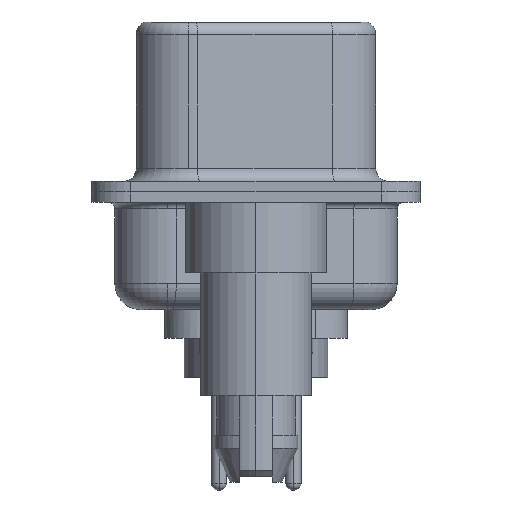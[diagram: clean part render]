
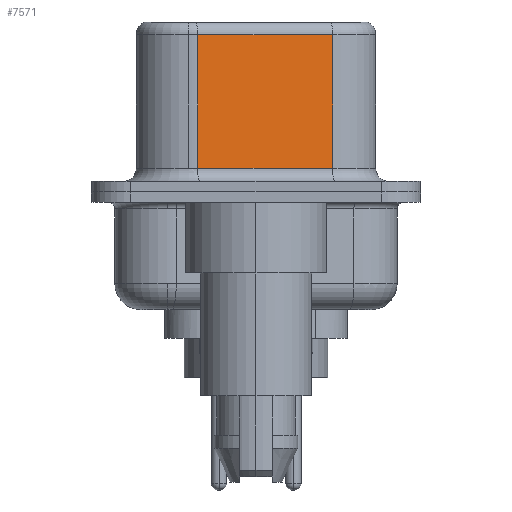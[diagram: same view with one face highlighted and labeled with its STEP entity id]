
A CAD part, left-side view. The second image highlights one B-rep face of the part: STEP entity #7571.
In plain terms, the highlighted planar face has unit normal (-0.985, -0.174, 0).
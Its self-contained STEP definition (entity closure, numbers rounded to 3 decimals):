
#718 = DIRECTION ( 'NONE',  ( 0., 0., -1. ) ) ;
#1950 = FACE_OUTER_BOUND ( 'NONE', #14733, .T. ) ;
#5108 = DIRECTION ( 'NONE',  ( -0.174, 0.985, 0. ) ) ;
#5463 = CARTESIAN_POINT ( 'NONE',  ( 4.58, -2.927, 0.9 ) ) ;
#5551 = CARTESIAN_POINT ( 'NONE',  ( 4.58, -2.927, 6.02 ) ) ;
#5612 = CARTESIAN_POINT ( 'NONE',  ( 4.58, -2.927, 6.02 ) ) ;
#6773 = VERTEX_POINT ( 'NONE', #5463 ) ;
#7039 = VERTEX_POINT ( 'NONE', #9002 ) ;
#7060 = DIRECTION ( 'NONE',  ( -0.174, 0.985, 0. ) ) ;
#7571 = ADVANCED_FACE ( 'NONE', ( #1950 ), #9399, .F. ) ;
#7811 = EDGE_CURVE ( 'NONE', #7039, #6773, #18312, .T. ) ;
#8519 = CARTESIAN_POINT ( 'NONE',  ( 3.67, 2.233, 6.52 ) ) ;
#9002 = CARTESIAN_POINT ( 'NONE',  ( 3.67, 2.233, 0.9 ) ) ;
#9286 = ORIENTED_EDGE ( 'NONE', *, *, #13643, .T. ) ;
#9399 = PLANE ( 'NONE',  #19000 ) ;
#9784 = ORIENTED_EDGE ( 'NONE', *, *, #12099, .F. ) ;
#9889 = DIRECTION ( 'NONE',  ( 0.174, -0.985, 0. ) ) ;
#10787 = ORIENTED_EDGE ( 'NONE', *, *, #7811, .T. ) ;
#10982 = CARTESIAN_POINT ( 'NONE',  ( 4.58, -2.927, 6.52 ) ) ;
#11325 = LINE ( 'NONE', #5612, #18797 ) ;
#11438 = VECTOR ( 'NONE', #17360, 1000. ) ;
#11714 = LINE ( 'NONE', #10982, #15245 ) ;
#11905 = LINE ( 'NONE', #8519, #11438 ) ;
#12099 = EDGE_CURVE ( 'NONE', #17632, #6773, #11714, .T. ) ;
#13347 = ORIENTED_EDGE ( 'NONE', *, *, #18717, .T. ) ;
#13643 = EDGE_CURVE ( 'NONE', #17560, #7039, #11905, .T. ) ;
#13933 = DIRECTION ( 'NONE',  ( 0.985, 0.174, 0. ) ) ;
#14363 = CARTESIAN_POINT ( 'NONE',  ( 4.58, -2.927, 0.9 ) ) ;
#14435 = VECTOR ( 'NONE', #9889, 1000. ) ;
#14733 = EDGE_LOOP ( 'NONE', ( #9784, #13347, #9286, #10787 ) ) ;
#15245 = VECTOR ( 'NONE', #718, 1000. ) ;
#15326 = CARTESIAN_POINT ( 'NONE',  ( 4.58, -2.927, 6.52 ) ) ;
#17360 = DIRECTION ( 'NONE',  ( 0., 0., -1. ) ) ;
#17560 = VERTEX_POINT ( 'NONE', #18664 ) ;
#17632 = VERTEX_POINT ( 'NONE', #5551 ) ;
#18312 = LINE ( 'NONE', #14363, #14435 ) ;
#18664 = CARTESIAN_POINT ( 'NONE',  ( 3.67, 2.233, 6.02 ) ) ;
#18717 = EDGE_CURVE ( 'NONE', #17632, #17560, #11325, .T. ) ;
#18797 = VECTOR ( 'NONE', #7060, 1000. ) ;
#19000 = AXIS2_PLACEMENT_3D ( 'NONE', #15326, #13933, #5108 ) ;
